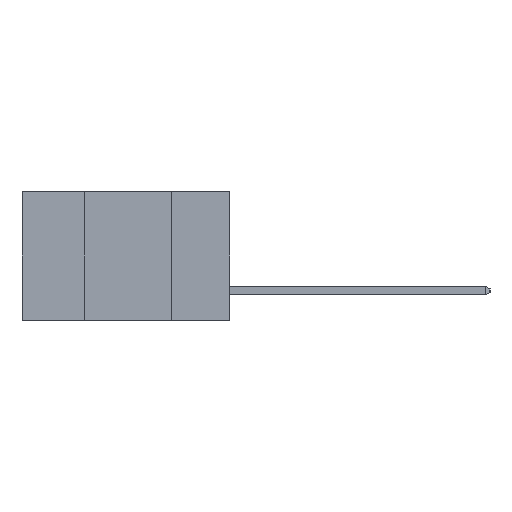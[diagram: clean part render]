
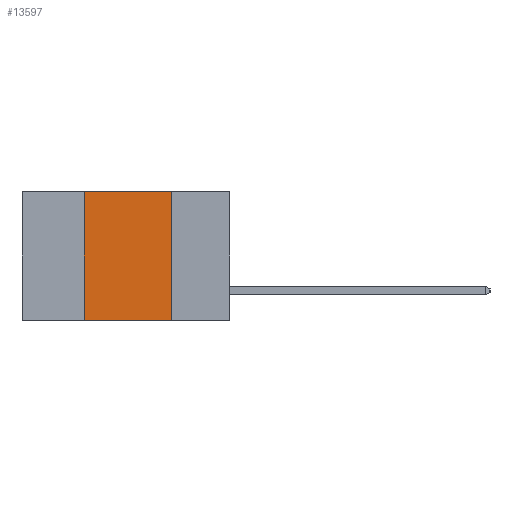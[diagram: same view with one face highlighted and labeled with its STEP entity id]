
A CAD part, left-side view. The second image highlights one B-rep face of the part: STEP entity #13597.
In plain terms, the highlighted planar face has unit normal (-1, 0, 0).
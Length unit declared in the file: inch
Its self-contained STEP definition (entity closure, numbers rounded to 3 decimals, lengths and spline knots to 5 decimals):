
#227 = EDGE_LOOP ( 'NONE', ( #10424, #3712, #13347, #10033 ) ) ;
#984 = EDGE_CURVE ( 'NONE', #12108, #14856, #10150, .T. ) ;
#2279 = VERTEX_POINT ( 'NONE', #3425 ) ;
#2398 = LINE ( 'NONE', #2683, #15404 ) ;
#2683 = CARTESIAN_POINT ( 'NONE',  ( 0., 0.6, 0. ) ) ;
#2921 = FACE_OUTER_BOUND ( 'NONE', #227, .T. ) ;
#3006 = EDGE_CURVE ( 'NONE', #12108, #2279, #14411, .T. ) ;
#3425 = CARTESIAN_POINT ( 'NONE',  ( 0., 0.17, -0.37 ) ) ;
#3534 = LINE ( 'NONE', #12614, #9871 ) ;
#3712 = ORIENTED_EDGE ( 'NONE', *, *, #10160, .F. ) ;
#4444 = VECTOR ( 'NONE', #4513, 39.37008 ) ;
#4513 = DIRECTION ( 'NONE',  ( 0., -1., 0. ) ) ;
#4904 = DIRECTION ( 'NONE',  ( 0., 0., 1. ) ) ;
#6969 = CARTESIAN_POINT ( 'NONE',  ( 0., 0.6, -0.37 ) ) ;
#7739 = CARTESIAN_POINT ( 'NONE',  ( 0., 0.42, -0.37 ) ) ;
#7811 = CARTESIAN_POINT ( 'NONE',  ( 0., 0.6, 0. ) ) ;
#8476 = CARTESIAN_POINT ( 'NONE',  ( 0., 0.17, 0. ) ) ;
#8924 = DIRECTION ( 'NONE',  ( 0., 0., -1. ) ) ;
#9071 = DIRECTION ( 'NONE',  ( 0., 0., -1. ) ) ;
#9340 = EDGE_CURVE ( 'NONE', #14167, #2279, #3534, .T. ) ;
#9462 = AXIS2_PLACEMENT_3D ( 'NONE', #7811, #16374, #9071 ) ;
#9871 = VECTOR ( 'NONE', #8924, 39.37008 ) ;
#10033 = ORIENTED_EDGE ( 'NONE', *, *, #3006, .T. ) ;
#10150 = LINE ( 'NONE', #14040, #15880 ) ;
#10160 = EDGE_CURVE ( 'NONE', #14856, #14167, #2398, .T. ) ;
#10424 = ORIENTED_EDGE ( 'NONE', *, *, #9340, .F. ) ;
#12108 = VERTEX_POINT ( 'NONE', #7739 ) ;
#12614 = CARTESIAN_POINT ( 'NONE',  ( 0., 0.17, -0.37 ) ) ;
#13347 = ORIENTED_EDGE ( 'NONE', *, *, #984, .F. ) ;
#13597 = ADVANCED_FACE ( 'NONE', ( #2921 ), #15194, .F. ) ;
#14040 = CARTESIAN_POINT ( 'NONE',  ( 0., 0.42, -0.37 ) ) ;
#14167 = VERTEX_POINT ( 'NONE', #8476 ) ;
#14411 = LINE ( 'NONE', #6969, #4444 ) ;
#14856 = VERTEX_POINT ( 'NONE', #15550 ) ;
#15194 = PLANE ( 'NONE',  #9462 ) ;
#15200 = DIRECTION ( 'NONE',  ( 0., -1., 0. ) ) ;
#15404 = VECTOR ( 'NONE', #15200, 39.37008 ) ;
#15550 = CARTESIAN_POINT ( 'NONE',  ( 0., 0.42, 0. ) ) ;
#15880 = VECTOR ( 'NONE', #4904, 39.37008 ) ;
#16374 = DIRECTION ( 'NONE',  ( 1., 0., 0. ) ) ;
